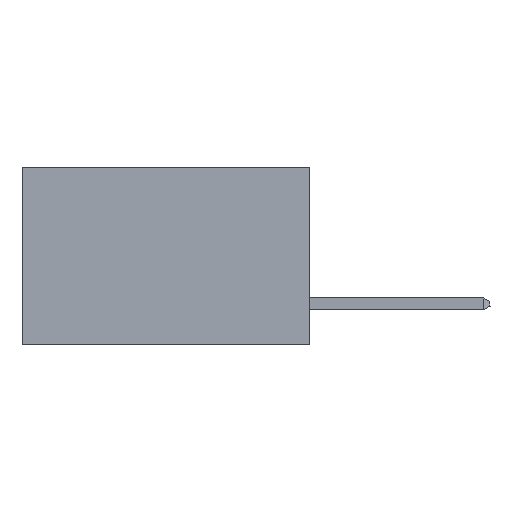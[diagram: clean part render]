
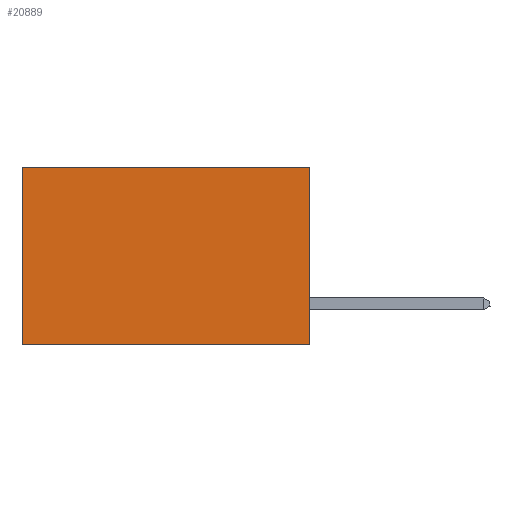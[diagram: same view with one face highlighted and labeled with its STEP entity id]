
A CAD part, left-side view. The second image highlights one B-rep face of the part: STEP entity #20889.
In plain terms, the highlighted planar face has unit normal (-1, 0, 0).
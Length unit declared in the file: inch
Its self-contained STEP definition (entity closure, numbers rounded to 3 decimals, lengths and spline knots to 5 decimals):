
#593 = CARTESIAN_POINT ( 'NONE',  ( 0.2875, 0., 0. ) ) ;
#1108 = DIRECTION ( 'NONE',  ( 0., 0., -1. ) ) ;
#2269 = ORIENTED_EDGE ( 'NONE', *, *, #15957, .F. ) ;
#2432 = CARTESIAN_POINT ( 'NONE',  ( 0.2875, 0., -0.37 ) ) ;
#2438 = ORIENTED_EDGE ( 'NONE', *, *, #3627, .T. ) ;
#3371 = CARTESIAN_POINT ( 'NONE',  ( 0.2875, 0.6, 0. ) ) ;
#3480 = DIRECTION ( 'NONE',  ( 0., 0., -1. ) ) ;
#3535 = VECTOR ( 'NONE', #3480, 39.37008 ) ;
#3627 = EDGE_CURVE ( 'NONE', #12354, #11203, #25992, .T. ) ;
#4583 = VECTOR ( 'NONE', #7427, 39.37008 ) ;
#5538 = DIRECTION ( 'NONE',  ( 0., 0., -1. ) ) ;
#5656 = ORIENTED_EDGE ( 'NONE', *, *, #14078, .T. ) ;
#7427 = DIRECTION ( 'NONE',  ( 0., 1., 0. ) ) ;
#7727 = PLANE ( 'NONE',  #22517 ) ;
#9559 = LINE ( 'NONE', #28460, #3535 ) ;
#10354 = LINE ( 'NONE', #18619, #14249 ) ;
#10660 = LINE ( 'NONE', #15076, #4583 ) ;
#11203 = VERTEX_POINT ( 'NONE', #3371 ) ;
#12354 = VERTEX_POINT ( 'NONE', #29225 ) ;
#12517 = DIRECTION ( 'NONE',  ( 1., 0., 0. ) ) ;
#14078 = EDGE_CURVE ( 'NONE', #11203, #19754, #9559, .T. ) ;
#14249 = VECTOR ( 'NONE', #1108, 39.37008 ) ;
#14486 = CARTESIAN_POINT ( 'NONE',  ( 0.2875, 0.6, -0.37 ) ) ;
#14717 = CARTESIAN_POINT ( 'NONE',  ( 0.2875, 0., 0. ) ) ;
#15076 = CARTESIAN_POINT ( 'NONE',  ( 0.2875, 0., -0.37 ) ) ;
#15957 = EDGE_CURVE ( 'NONE', #21313, #19754, #10660, .T. ) ;
#16447 = VECTOR ( 'NONE', #21012, 39.37008 ) ;
#18305 = EDGE_LOOP ( 'NONE', ( #5656, #2269, #22419, #2438 ) ) ;
#18619 = CARTESIAN_POINT ( 'NONE',  ( 0.2875, 0., 0. ) ) ;
#19754 = VERTEX_POINT ( 'NONE', #14486 ) ;
#20889 = ADVANCED_FACE ( 'NONE', ( #23795 ), #7727, .F. ) ;
#21012 = DIRECTION ( 'NONE',  ( 0., 1., 0. ) ) ;
#21313 = VERTEX_POINT ( 'NONE', #2432 ) ;
#22419 = ORIENTED_EDGE ( 'NONE', *, *, #29304, .F. ) ;
#22517 = AXIS2_PLACEMENT_3D ( 'NONE', #14717, #12517, #5538 ) ;
#23795 = FACE_OUTER_BOUND ( 'NONE', #18305, .T. ) ;
#25992 = LINE ( 'NONE', #593, #16447 ) ;
#28460 = CARTESIAN_POINT ( 'NONE',  ( 0.2875, 0.6, 0. ) ) ;
#29225 = CARTESIAN_POINT ( 'NONE',  ( 0.2875, 0., 0. ) ) ;
#29304 = EDGE_CURVE ( 'NONE', #12354, #21313, #10354, .T. ) ;
